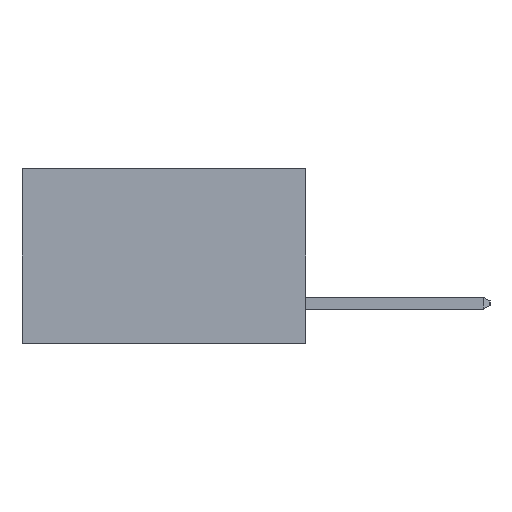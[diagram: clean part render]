
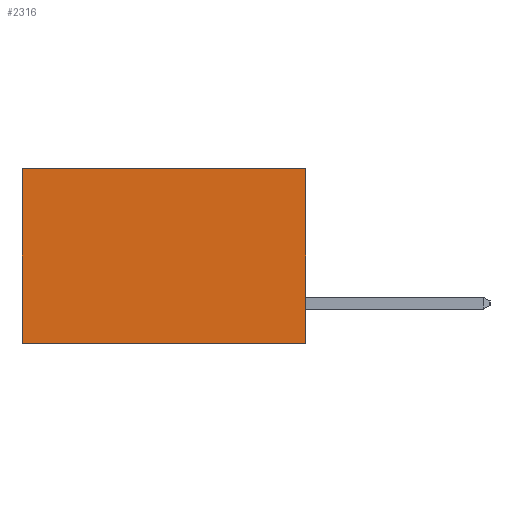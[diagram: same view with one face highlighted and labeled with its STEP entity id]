
A CAD part, left-side view. The second image highlights one B-rep face of the part: STEP entity #2316.
In plain terms, the highlighted planar face has unit normal (-1, 0, 0).
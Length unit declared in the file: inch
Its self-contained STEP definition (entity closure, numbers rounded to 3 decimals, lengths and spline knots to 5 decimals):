
#380 = EDGE_CURVE ( 'NONE', #2185, #9951, #7367, .T. ) ;
#978 = ORIENTED_EDGE ( 'NONE', *, *, #17941, .F. ) ;
#1133 = DIRECTION ( 'NONE',  ( 0., 0., -1. ) ) ;
#2185 = VERTEX_POINT ( 'NONE', #4229 ) ;
#2298 = LINE ( 'NONE', #13871, #5622 ) ;
#2316 = ADVANCED_FACE ( 'NONE', ( #6888 ), #15540, .F. ) ;
#4229 = CARTESIAN_POINT ( 'NONE',  ( 0.298, 0., 0. ) ) ;
#4705 = DIRECTION ( 'NONE',  ( 0., 0., -1. ) ) ;
#4831 = VERTEX_POINT ( 'NONE', #14220 ) ;
#5124 = DIRECTION ( 'NONE',  ( 0., 1., 0. ) ) ;
#5622 = VECTOR ( 'NONE', #1133, 39.37008 ) ;
#6301 = VECTOR ( 'NONE', #10038, 39.37008 ) ;
#6888 = FACE_OUTER_BOUND ( 'NONE', #10545, .T. ) ;
#7034 = VERTEX_POINT ( 'NONE', #7737 ) ;
#7268 = LINE ( 'NONE', #11823, #10631 ) ;
#7367 = LINE ( 'NONE', #8336, #14877 ) ;
#7608 = LINE ( 'NONE', #16957, #6301 ) ;
#7737 = CARTESIAN_POINT ( 'NONE',  ( 0.298, 0., -0.37 ) ) ;
#8336 = CARTESIAN_POINT ( 'NONE',  ( 0.298, 0., 0. ) ) ;
#9951 = VERTEX_POINT ( 'NONE', #15335 ) ;
#10038 = DIRECTION ( 'NONE',  ( 0., 1., 0. ) ) ;
#10545 = EDGE_LOOP ( 'NONE', ( #12949, #14670, #978, #16811 ) ) ;
#10631 = VECTOR ( 'NONE', #4705, 39.37008 ) ;
#10889 = DIRECTION ( 'NONE',  ( 0., 0., -1. ) ) ;
#11245 = DIRECTION ( 'NONE',  ( 1., 0., 0. ) ) ;
#11823 = CARTESIAN_POINT ( 'NONE',  ( 0.298, 0.6, 0. ) ) ;
#12509 = EDGE_CURVE ( 'NONE', #7034, #4831, #7608, .T. ) ;
#12949 = ORIENTED_EDGE ( 'NONE', *, *, #16201, .T. ) ;
#13572 = AXIS2_PLACEMENT_3D ( 'NONE', #15308, #11245, #10889 ) ;
#13871 = CARTESIAN_POINT ( 'NONE',  ( 0.298, 0., 0. ) ) ;
#14220 = CARTESIAN_POINT ( 'NONE',  ( 0.298, 0.6, -0.37 ) ) ;
#14670 = ORIENTED_EDGE ( 'NONE', *, *, #12509, .F. ) ;
#14877 = VECTOR ( 'NONE', #5124, 39.37008 ) ;
#15308 = CARTESIAN_POINT ( 'NONE',  ( 0.298, 0., 0. ) ) ;
#15335 = CARTESIAN_POINT ( 'NONE',  ( 0.298, 0.6, 0. ) ) ;
#15540 = PLANE ( 'NONE',  #13572 ) ;
#16201 = EDGE_CURVE ( 'NONE', #9951, #4831, #7268, .T. ) ;
#16811 = ORIENTED_EDGE ( 'NONE', *, *, #380, .T. ) ;
#16957 = CARTESIAN_POINT ( 'NONE',  ( 0.298, 0., -0.37 ) ) ;
#17941 = EDGE_CURVE ( 'NONE', #2185, #7034, #2298, .T. ) ;
